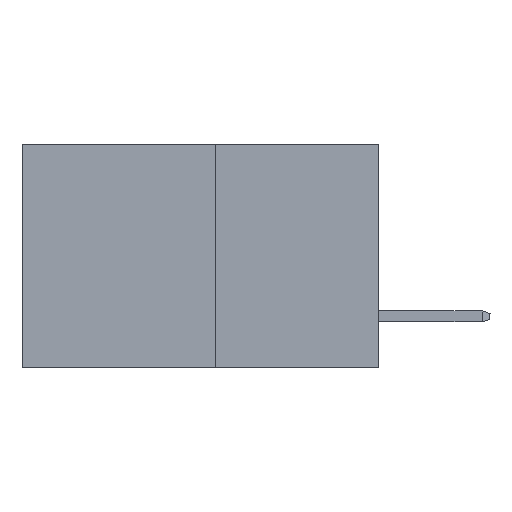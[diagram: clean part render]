
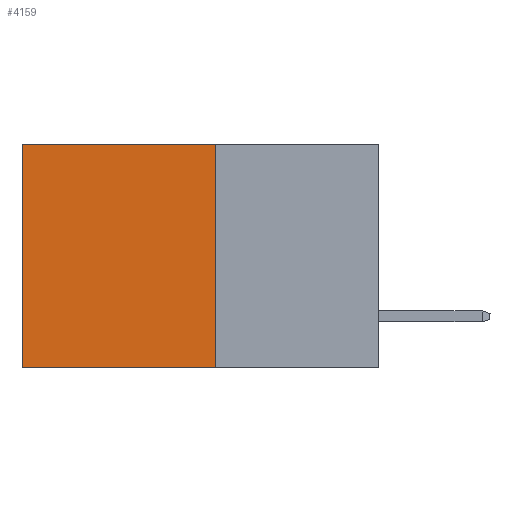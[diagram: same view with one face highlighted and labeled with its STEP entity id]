
A CAD part, left-side view. The second image highlights one B-rep face of the part: STEP entity #4159.
In plain terms, the highlighted planar face has unit normal (-1, 0, 0).
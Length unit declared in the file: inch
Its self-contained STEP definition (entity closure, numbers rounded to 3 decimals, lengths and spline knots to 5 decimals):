
#153 = ORIENTED_EDGE ( 'NONE', *, *, #9672, .T. ) ;
#315 = CARTESIAN_POINT ( 'NONE',  ( 0.277, 0.27, -0.37 ) ) ;
#393 = ORIENTED_EDGE ( 'NONE', *, *, #13097, .F. ) ;
#1989 = LINE ( 'NONE', #315, #2435 ) ;
#2435 = VECTOR ( 'NONE', #10037, 39.37008 ) ;
#3833 = LINE ( 'NONE', #16480, #4257 ) ;
#4159 = ADVANCED_FACE ( 'NONE', ( #8436 ), #7547, .F. ) ;
#4257 = VECTOR ( 'NONE', #7168, 39.37008 ) ;
#4315 = CARTESIAN_POINT ( 'NONE',  ( 0.277, 0.59, 0. ) ) ;
#4731 = VECTOR ( 'NONE', #16906, 39.37008 ) ;
#5460 = ORIENTED_EDGE ( 'NONE', *, *, #14470, .F. ) ;
#6225 = AXIS2_PLACEMENT_3D ( 'NONE', #7612, #6609, #6384 ) ;
#6347 = VERTEX_POINT ( 'NONE', #4315 ) ;
#6384 = DIRECTION ( 'NONE',  ( 0., 0., -1. ) ) ;
#6534 = VERTEX_POINT ( 'NONE', #17149 ) ;
#6609 = DIRECTION ( 'NONE',  ( 1., 0., 0. ) ) ;
#7145 = CARTESIAN_POINT ( 'NONE',  ( 0.277, 0.27, -0.37 ) ) ;
#7168 = DIRECTION ( 'NONE',  ( 0., 1., 0. ) ) ;
#7481 = EDGE_LOOP ( 'NONE', ( #153, #393, #5460, #17074 ) ) ;
#7547 = PLANE ( 'NONE',  #6225 ) ;
#7612 = CARTESIAN_POINT ( 'NONE',  ( 0.277, 0.27, -0.37 ) ) ;
#7622 = CARTESIAN_POINT ( 'NONE',  ( 0.277, 0.59, -0.37 ) ) ;
#7824 = CARTESIAN_POINT ( 'NONE',  ( 0.277, 0.59, -0.37 ) ) ;
#8436 = FACE_OUTER_BOUND ( 'NONE', #7481, .T. ) ;
#8463 = LINE ( 'NONE', #7622, #4731 ) ;
#9064 = CARTESIAN_POINT ( 'NONE',  ( 0.277, 0.27, 0. ) ) ;
#9150 = VERTEX_POINT ( 'NONE', #7824 ) ;
#9672 = EDGE_CURVE ( 'NONE', #6347, #9150, #8463, .T. ) ;
#10037 = DIRECTION ( 'NONE',  ( 0., 0., -1. ) ) ;
#13097 = EDGE_CURVE ( 'NONE', #13749, #9150, #3833, .T. ) ;
#13749 = VERTEX_POINT ( 'NONE', #7145 ) ;
#13978 = LINE ( 'NONE', #9064, #16661 ) ;
#14470 = EDGE_CURVE ( 'NONE', #6534, #13749, #1989, .T. ) ;
#14649 = EDGE_CURVE ( 'NONE', #6534, #6347, #13978, .T. ) ;
#16480 = CARTESIAN_POINT ( 'NONE',  ( 0.277, 0.27, -0.37 ) ) ;
#16661 = VECTOR ( 'NONE', #17003, 39.37008 ) ;
#16906 = DIRECTION ( 'NONE',  ( 0., 0., -1. ) ) ;
#17003 = DIRECTION ( 'NONE',  ( 0., 1., 0. ) ) ;
#17074 = ORIENTED_EDGE ( 'NONE', *, *, #14649, .T. ) ;
#17149 = CARTESIAN_POINT ( 'NONE',  ( 0.277, 0.27, 0. ) ) ;
